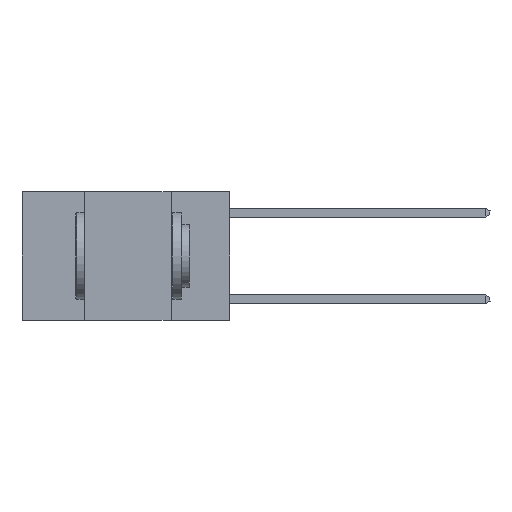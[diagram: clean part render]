
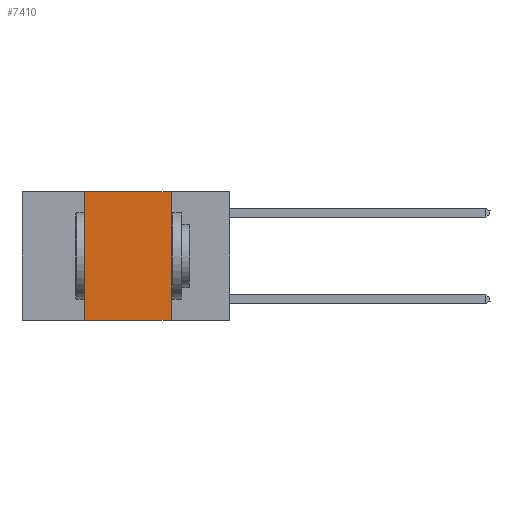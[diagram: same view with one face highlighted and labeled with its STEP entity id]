
A CAD part, left-side view. The second image highlights one B-rep face of the part: STEP entity #7410.
In plain terms, the highlighted planar face has unit normal (-1, 0, 0).
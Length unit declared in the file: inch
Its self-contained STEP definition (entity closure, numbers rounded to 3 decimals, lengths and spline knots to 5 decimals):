
#78 = EDGE_CURVE ( 'NONE', #1713, #13179, #1663, .T. ) ;
#448 = DIRECTION ( 'NONE',  ( 0., 0., 1. ) ) ;
#586 = LINE ( 'NONE', #9642, #10853 ) ;
#893 = DIRECTION ( 'NONE',  ( 1., 0., 0. ) ) ;
#1663 = LINE ( 'NONE', #8507, #7469 ) ;
#1713 = VERTEX_POINT ( 'NONE', #8428 ) ;
#1851 = PLANE ( 'NONE',  #13525 ) ;
#2326 = EDGE_CURVE ( 'NONE', #11783, #1713, #586, .T. ) ;
#2844 = DIRECTION ( 'NONE',  ( 0., -1., 0. ) ) ;
#3446 = ORIENTED_EDGE ( 'NONE', *, *, #2326, .F. ) ;
#4560 = ORIENTED_EDGE ( 'NONE', *, *, #13273, .F. ) ;
#4590 = CARTESIAN_POINT ( 'NONE',  ( 0., 0.6, -0.37 ) ) ;
#5034 = CARTESIAN_POINT ( 'NONE',  ( 0., 0.17, 0. ) ) ;
#5996 = VECTOR ( 'NONE', #14098, 39.37008 ) ;
#6245 = ORIENTED_EDGE ( 'NONE', *, *, #78, .F. ) ;
#7410 = ADVANCED_FACE ( 'NONE', ( #8696 ), #1851, .F. ) ;
#7469 = VECTOR ( 'NONE', #2844, 39.37008 ) ;
#8005 = VERTEX_POINT ( 'NONE', #9689 ) ;
#8104 = DIRECTION ( 'NONE',  ( 0., -1., 0. ) ) ;
#8428 = CARTESIAN_POINT ( 'NONE',  ( 0., 0.42, 0. ) ) ;
#8507 = CARTESIAN_POINT ( 'NONE',  ( 0., 0.6, 0. ) ) ;
#8680 = LINE ( 'NONE', #5034, #5996 ) ;
#8696 = FACE_OUTER_BOUND ( 'NONE', #10500, .T. ) ;
#8990 = CARTESIAN_POINT ( 'NONE',  ( 0., 0.42, -0.37 ) ) ;
#9318 = VECTOR ( 'NONE', #8104, 39.37008 ) ;
#9642 = CARTESIAN_POINT ( 'NONE',  ( 0., 0.42, 0. ) ) ;
#9689 = CARTESIAN_POINT ( 'NONE',  ( 0., 0.17, -0.37 ) ) ;
#9787 = ORIENTED_EDGE ( 'NONE', *, *, #14032, .T. ) ;
#10399 = LINE ( 'NONE', #4590, #9318 ) ;
#10500 = EDGE_LOOP ( 'NONE', ( #4560, #6245, #3446, #9787 ) ) ;
#10853 = VECTOR ( 'NONE', #448, 39.37008 ) ;
#11783 = VERTEX_POINT ( 'NONE', #8990 ) ;
#13179 = VERTEX_POINT ( 'NONE', #13808 ) ;
#13273 = EDGE_CURVE ( 'NONE', #13179, #8005, #8680, .T. ) ;
#13525 = AXIS2_PLACEMENT_3D ( 'NONE', #14548, #893, #14415 ) ;
#13808 = CARTESIAN_POINT ( 'NONE',  ( 0., 0.17, 0. ) ) ;
#14032 = EDGE_CURVE ( 'NONE', #11783, #8005, #10399, .T. ) ;
#14098 = DIRECTION ( 'NONE',  ( 0., 0., -1. ) ) ;
#14415 = DIRECTION ( 'NONE',  ( 0., 0., -1. ) ) ;
#14548 = CARTESIAN_POINT ( 'NONE',  ( 0., 0.6, 0. ) ) ;
